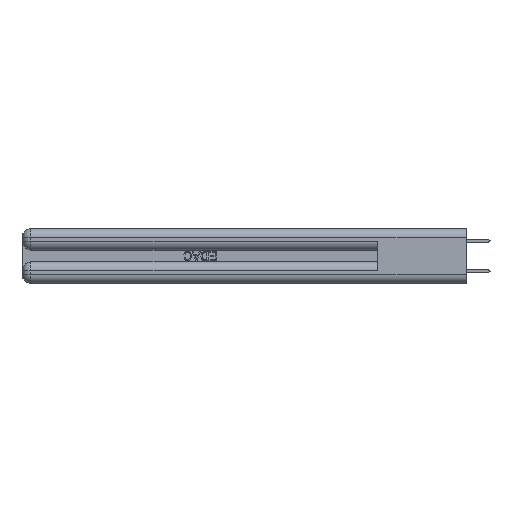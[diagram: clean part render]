
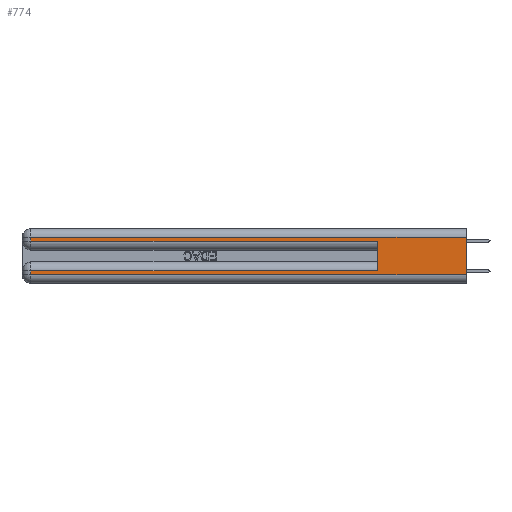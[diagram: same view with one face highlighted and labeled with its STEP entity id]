
A CAD part, left-side view. The second image highlights one B-rep face of the part: STEP entity #774.
In plain terms, the highlighted planar face has unit normal (-1, 0, 0).
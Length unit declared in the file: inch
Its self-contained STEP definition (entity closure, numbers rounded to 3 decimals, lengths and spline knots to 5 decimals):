
#628 = AXIS2_PLACEMENT_3D ( 'NONE', #5418, #12502, #36945 ) ;
#774 = ADVANCED_FACE ( 'NONE', ( #10475 ), #33409, .F. ) ;
#824 = VERTEX_POINT ( 'NONE', #22951 ) ;
#2323 = ORIENTED_EDGE ( 'NONE', *, *, #19810, .F. ) ;
#2588 = CARTESIAN_POINT ( 'NONE',  ( 0., 0., 0.31 ) ) ;
#3406 = DIRECTION ( 'NONE',  ( 0., -1., 0. ) ) ;
#3699 = LINE ( 'NONE', #13008, #11978 ) ;
#4855 = VERTEX_POINT ( 'NONE', #8976 ) ;
#5418 = CARTESIAN_POINT ( 'NONE',  ( 0., 0., 0.37 ) ) ;
#5592 = CARTESIAN_POINT ( 'NONE',  ( 0., 2.94, 0.06 ) ) ;
#6183 = DIRECTION ( 'NONE',  ( 0., 1., 0. ) ) ;
#7586 = EDGE_CURVE ( 'NONE', #4855, #44060, #15262, .T. ) ;
#7587 = EDGE_CURVE ( 'NONE', #42837, #22441, #3699, .T. ) ;
#7871 = EDGE_CURVE ( 'NONE', #22858, #19302, #11426, .T. ) ;
#8572 = VECTOR ( 'NONE', #33084, 39.37008 ) ;
#8638 = CARTESIAN_POINT ( 'NONE',  ( 0., 0.6, 0.145 ) ) ;
#8976 = CARTESIAN_POINT ( 'NONE',  ( 0., 2.94, 0.285 ) ) ;
#8988 = ORIENTED_EDGE ( 'NONE', *, *, #23627, .T. ) ;
#9873 = VECTOR ( 'NONE', #6183, 39.37008 ) ;
#10475 = FACE_OUTER_BOUND ( 'NONE', #18852, .T. ) ;
#10780 = ORIENTED_EDGE ( 'NONE', *, *, #33016, .T. ) ;
#10973 = LINE ( 'NONE', #2588, #9873 ) ;
#11426 = LINE ( 'NONE', #18028, #28875 ) ;
#11978 = VECTOR ( 'NONE', #27006, 39.37008 ) ;
#12502 = DIRECTION ( 'NONE',  ( 1., 0., 0. ) ) ;
#12685 = CARTESIAN_POINT ( 'NONE',  ( 0., 2.94, 0.085 ) ) ;
#13008 = CARTESIAN_POINT ( 'NONE',  ( 0., 0., 0.37 ) ) ;
#13911 = CARTESIAN_POINT ( 'NONE',  ( 0., 0., 0.06 ) ) ;
#13993 = LINE ( 'NONE', #22554, #22088 ) ;
#14260 = CARTESIAN_POINT ( 'NONE',  ( 0., 0.6, 0.285 ) ) ;
#15262 = LINE ( 'NONE', #23301, #30546 ) ;
#16330 = ORIENTED_EDGE ( 'NONE', *, *, #7871, .T. ) ;
#16787 = LINE ( 'NONE', #8638, #8572 ) ;
#18028 = CARTESIAN_POINT ( 'NONE',  ( 0., 2.94, 0.37 ) ) ;
#18852 = EDGE_LOOP ( 'NONE', ( #19950, #8988, #38848, #35102, #2323, #10780, #16330, #26399 ) ) ;
#19302 = VERTEX_POINT ( 'NONE', #5592 ) ;
#19666 = CARTESIAN_POINT ( 'NONE',  ( 0., 0., 0.085 ) ) ;
#19810 = EDGE_CURVE ( 'NONE', #38892, #44060, #16787, .T. ) ;
#19950 = ORIENTED_EDGE ( 'NONE', *, *, #7587, .F. ) ;
#22088 = VECTOR ( 'NONE', #29803, 39.37008 ) ;
#22441 = VERTEX_POINT ( 'NONE', #13911 ) ;
#22451 = EDGE_CURVE ( 'NONE', #19302, #22441, #36201, .T. ) ;
#22554 = CARTESIAN_POINT ( 'NONE',  ( 0., 2.94, 0.37 ) ) ;
#22858 = VERTEX_POINT ( 'NONE', #12685 ) ;
#22951 = CARTESIAN_POINT ( 'NONE',  ( 0., 2.94, 0.31 ) ) ;
#23301 = CARTESIAN_POINT ( 'NONE',  ( 0., 0., 0.285 ) ) ;
#23627 = EDGE_CURVE ( 'NONE', #42837, #824, #10973, .T. ) ;
#23942 = VECTOR ( 'NONE', #44102, 39.37008 ) ;
#26399 = ORIENTED_EDGE ( 'NONE', *, *, #22451, .T. ) ;
#27006 = DIRECTION ( 'NONE',  ( 0., 0., -1. ) ) ;
#28875 = VECTOR ( 'NONE', #35433, 39.37008 ) ;
#29803 = DIRECTION ( 'NONE',  ( 0., 0., -1. ) ) ;
#30546 = VECTOR ( 'NONE', #44440, 39.37008 ) ;
#32206 = LINE ( 'NONE', #19666, #23942 ) ;
#33016 = EDGE_CURVE ( 'NONE', #38892, #22858, #32206, .T. ) ;
#33084 = DIRECTION ( 'NONE',  ( 0., 0., 1. ) ) ;
#33409 = PLANE ( 'NONE',  #628 ) ;
#35102 = ORIENTED_EDGE ( 'NONE', *, *, #7586, .T. ) ;
#35149 = EDGE_CURVE ( 'NONE', #824, #4855, #13993, .T. ) ;
#35433 = DIRECTION ( 'NONE',  ( 0., 0., -1. ) ) ;
#36201 = LINE ( 'NONE', #38364, #37314 ) ;
#36945 = DIRECTION ( 'NONE',  ( 0., 0., -1. ) ) ;
#37314 = VECTOR ( 'NONE', #3406, 39.37008 ) ;
#38364 = CARTESIAN_POINT ( 'NONE',  ( 0., 0., 0.06 ) ) ;
#38848 = ORIENTED_EDGE ( 'NONE', *, *, #35149, .T. ) ;
#38892 = VERTEX_POINT ( 'NONE', #42960 ) ;
#40243 = CARTESIAN_POINT ( 'NONE',  ( 0., 0., 0.31 ) ) ;
#42837 = VERTEX_POINT ( 'NONE', #40243 ) ;
#42960 = CARTESIAN_POINT ( 'NONE',  ( 0., 0.6, 0.085 ) ) ;
#44060 = VERTEX_POINT ( 'NONE', #14260 ) ;
#44102 = DIRECTION ( 'NONE',  ( 0., 1., 0. ) ) ;
#44440 = DIRECTION ( 'NONE',  ( 0., -1., 0. ) ) ;
